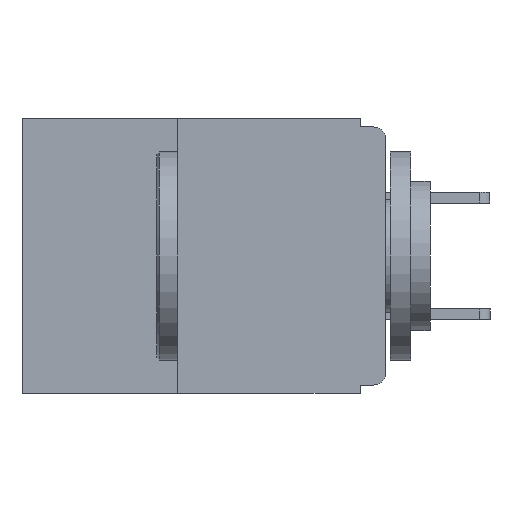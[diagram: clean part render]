
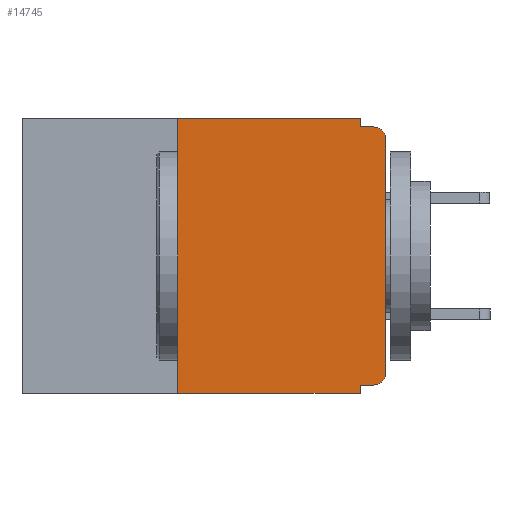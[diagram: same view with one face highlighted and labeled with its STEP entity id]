
A CAD part, left-side view. The second image highlights one B-rep face of the part: STEP entity #14745.
In plain terms, the highlighted planar face has unit normal (-1, 0, 0).
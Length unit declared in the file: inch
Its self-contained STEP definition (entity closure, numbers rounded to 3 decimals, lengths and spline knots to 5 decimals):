
#196 = EDGE_CURVE ( 'NONE', #5865, #3438, #9978, .T. ) ;
#361 = LINE ( 'NONE', #1975, #11398 ) ;
#576 = EDGE_CURVE ( 'NONE', #5759, #5865, #1336, .T. ) ;
#882 = ORIENTED_EDGE ( 'NONE', *, *, #7645, .F. ) ;
#1022 = VECTOR ( 'NONE', #7794, 39.37008 ) ;
#1269 = CARTESIAN_POINT ( 'NONE',  ( 0., 0., -0.025 ) ) ;
#1336 = LINE ( 'NONE', #15100, #14066 ) ;
#1773 = CARTESIAN_POINT ( 'NONE',  ( 0., 0., -0.305 ) ) ;
#1975 = CARTESIAN_POINT ( 'NONE',  ( 0., 0., 0. ) ) ;
#1993 = DIRECTION ( 'NONE',  ( 1., 0., 0. ) ) ;
#2052 = DIRECTION ( 'NONE',  ( 0., 0., 1. ) ) ;
#2471 = DIRECTION ( 'NONE',  ( 0., 0., -1. ) ) ;
#2721 = CARTESIAN_POINT ( 'NONE',  ( 0., 0.015, -0.32 ) ) ;
#3036 = AXIS2_PLACEMENT_3D ( 'NONE', #8070, #11432, #11348 ) ;
#3067 = VERTEX_POINT ( 'NONE', #1269 ) ;
#3438 = VERTEX_POINT ( 'NONE', #16263 ) ;
#3445 = CARTESIAN_POINT ( 'NONE',  ( 0., 0.031, 0. ) ) ;
#3474 = CARTESIAN_POINT ( 'NONE',  ( 0., 0.437, 0. ) ) ;
#3502 = ORIENTED_EDGE ( 'NONE', *, *, #10378, .T. ) ;
#3510 = DIRECTION ( 'NONE',  ( 0., -1., 0. ) ) ;
#3655 = VECTOR ( 'NONE', #14759, 39.37008 ) ;
#4539 = LINE ( 'NONE', #7867, #1022 ) ;
#4591 = EDGE_CURVE ( 'NONE', #4803, #10051, #10015, .T. ) ;
#4615 = ORIENTED_EDGE ( 'NONE', *, *, #9711, .F. ) ;
#4803 = VERTEX_POINT ( 'NONE', #7611 ) ;
#5001 = ORIENTED_EDGE ( 'NONE', *, *, #4591, .F. ) ;
#5046 = VECTOR ( 'NONE', #3510, 39.37008 ) ;
#5061 = ORIENTED_EDGE ( 'NONE', *, *, #8090, .T. ) ;
#5137 = CARTESIAN_POINT ( 'NONE',  ( 0., 0.015, -0.01 ) ) ;
#5197 = VERTEX_POINT ( 'NONE', #3445 ) ;
#5227 = ORIENTED_EDGE ( 'NONE', *, *, #196, .F. ) ;
#5354 = EDGE_CURVE ( 'NONE', #3067, #10051, #16322, .T. ) ;
#5444 = EDGE_CURVE ( 'NONE', #5759, #13193, #11166, .T. ) ;
#5668 = ORIENTED_EDGE ( 'NONE', *, *, #576, .F. ) ;
#5727 = ORIENTED_EDGE ( 'NONE', *, *, #5444, .T. ) ;
#5759 = VERTEX_POINT ( 'NONE', #2721 ) ;
#5865 = VERTEX_POINT ( 'NONE', #12386 ) ;
#5952 = EDGE_LOOP ( 'NONE', ( #3502, #6370, #5001, #6731, #882, #4615, #5061, #5227, #5668, #5727 ) ) ;
#6370 = ORIENTED_EDGE ( 'NONE', *, *, #5354, .T. ) ;
#6731 = ORIENTED_EDGE ( 'NONE', *, *, #12236, .F. ) ;
#6927 = DIRECTION ( 'NONE',  ( 0., 0., -1. ) ) ;
#7211 = PLANE ( 'NONE',  #8411 ) ;
#7558 = CARTESIAN_POINT ( 'NONE',  ( 0., 0.031, -0.33 ) ) ;
#7570 = CARTESIAN_POINT ( 'NONE',  ( 0., 0.25, 0. ) ) ;
#7611 = CARTESIAN_POINT ( 'NONE',  ( 0., 0.031, -0.01 ) ) ;
#7645 = EDGE_CURVE ( 'NONE', #12173, #5197, #14968, .T. ) ;
#7794 = DIRECTION ( 'NONE',  ( 0., 0., 1. ) ) ;
#7867 = CARTESIAN_POINT ( 'NONE',  ( 0., 0.25, -0.33 ) ) ;
#8070 = CARTESIAN_POINT ( 'NONE',  ( 0., 0.015, -0.025 ) ) ;
#8090 = EDGE_CURVE ( 'NONE', #14085, #3438, #11700, .T. ) ;
#8260 = AXIS2_PLACEMENT_3D ( 'NONE', #9474, #9113, #13487 ) ;
#8411 = AXIS2_PLACEMENT_3D ( 'NONE', #9698, #1993, #10934 ) ;
#9113 = DIRECTION ( 'NONE',  ( -1., 0., 0. ) ) ;
#9136 = FACE_OUTER_BOUND ( 'NONE', #5952, .T. ) ;
#9474 = CARTESIAN_POINT ( 'NONE',  ( 0., 0.015, -0.305 ) ) ;
#9609 = VECTOR ( 'NONE', #6927, 39.37008 ) ;
#9698 = CARTESIAN_POINT ( 'NONE',  ( 0., 0.437, 0. ) ) ;
#9711 = EDGE_CURVE ( 'NONE', #14085, #12173, #4539, .T. ) ;
#9978 = LINE ( 'NONE', #7558, #9609 ) ;
#10015 = LINE ( 'NONE', #14780, #3655 ) ;
#10051 = VERTEX_POINT ( 'NONE', #5137 ) ;
#10137 = CARTESIAN_POINT ( 'NONE',  ( 0., 0.031, 0. ) ) ;
#10153 = VECTOR ( 'NONE', #2471, 39.37008 ) ;
#10378 = EDGE_CURVE ( 'NONE', #13193, #3067, #361, .T. ) ;
#10934 = DIRECTION ( 'NONE',  ( 0., 0., -1. ) ) ;
#11166 = CIRCLE ( 'NONE', #8260, 0.015 ) ;
#11348 = DIRECTION ( 'NONE',  ( 0., 0., -1. ) ) ;
#11398 = VECTOR ( 'NONE', #2052, 39.37008 ) ;
#11432 = DIRECTION ( 'NONE',  ( -1., 0., 0. ) ) ;
#11686 = DIRECTION ( 'NONE',  ( 0., -1., 0. ) ) ;
#11700 = LINE ( 'NONE', #11722, #14575 ) ;
#11722 = CARTESIAN_POINT ( 'NONE',  ( 0., 0.437, -0.33 ) ) ;
#12004 = CARTESIAN_POINT ( 'NONE',  ( 0., 0.25, -0.33 ) ) ;
#12173 = VERTEX_POINT ( 'NONE', #7570 ) ;
#12236 = EDGE_CURVE ( 'NONE', #5197, #4803, #13514, .T. ) ;
#12386 = CARTESIAN_POINT ( 'NONE',  ( 0., 0.031, -0.32 ) ) ;
#12733 = DIRECTION ( 'NONE',  ( 0., 1., 0. ) ) ;
#13193 = VERTEX_POINT ( 'NONE', #1773 ) ;
#13487 = DIRECTION ( 'NONE',  ( 0., 0., -1. ) ) ;
#13514 = LINE ( 'NONE', #10137, #10153 ) ;
#14066 = VECTOR ( 'NONE', #12733, 39.37008 ) ;
#14085 = VERTEX_POINT ( 'NONE', #12004 ) ;
#14575 = VECTOR ( 'NONE', #11686, 39.37008 ) ;
#14745 = ADVANCED_FACE ( 'NONE', ( #9136 ), #7211, .F. ) ;
#14759 = DIRECTION ( 'NONE',  ( 0., -1., 0. ) ) ;
#14780 = CARTESIAN_POINT ( 'NONE',  ( 0., 0., -0.01 ) ) ;
#14968 = LINE ( 'NONE', #3474, #5046 ) ;
#15100 = CARTESIAN_POINT ( 'NONE',  ( 0., 0., -0.32 ) ) ;
#16263 = CARTESIAN_POINT ( 'NONE',  ( 0., 0.031, -0.33 ) ) ;
#16322 = CIRCLE ( 'NONE', #3036, 0.015 ) ;
